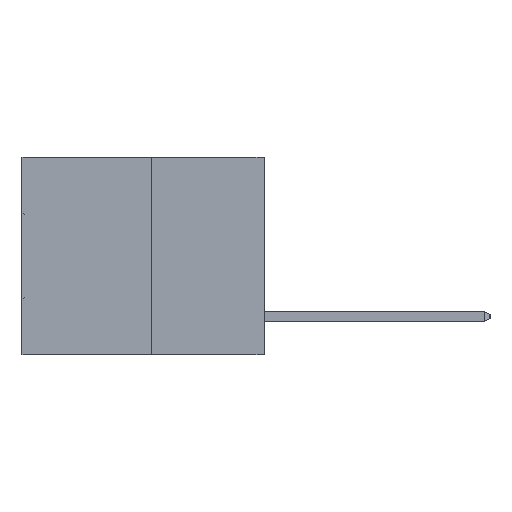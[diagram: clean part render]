
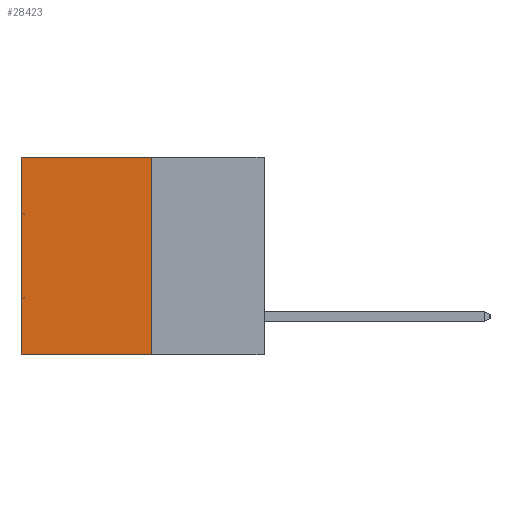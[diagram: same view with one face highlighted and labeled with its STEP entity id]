
A CAD part, left-side view. The second image highlights one B-rep face of the part: STEP entity #28423.
In plain terms, the highlighted planar face has unit normal (-1, 0, 0).
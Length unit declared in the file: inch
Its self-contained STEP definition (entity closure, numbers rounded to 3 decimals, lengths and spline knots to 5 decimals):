
#1631 = ORIENTED_EDGE ( 'NONE', *, *, #28231, .F. ) ;
#2117 = VERTEX_POINT ( 'NONE', #7423 ) ;
#2486 = CARTESIAN_POINT ( 'NONE',  ( 0.3165, 0.6, 0. ) ) ;
#2549 = CARTESIAN_POINT ( 'NONE',  ( 0.3165, 0.28, -0.49 ) ) ;
#2918 = CARTESIAN_POINT ( 'NONE',  ( 0.3165, 0.28, -0.49 ) ) ;
#4837 = LINE ( 'NONE', #11628, #22365 ) ;
#5639 = ORIENTED_EDGE ( 'NONE', *, *, #14806, .T. ) ;
#6487 = CARTESIAN_POINT ( 'NONE',  ( 0.3165, 0.6, -0.49 ) ) ;
#7120 = AXIS2_PLACEMENT_3D ( 'NONE', #2549, #17815, #20364 ) ;
#7423 = CARTESIAN_POINT ( 'NONE',  ( 0.3165, 0.28, 0. ) ) ;
#8020 = EDGE_CURVE ( 'NONE', #2117, #30886, #32022, .T. ) ;
#8221 = VERTEX_POINT ( 'NONE', #16242 ) ;
#10411 = DIRECTION ( 'NONE',  ( 0., 1., 0. ) ) ;
#11049 = VECTOR ( 'NONE', #24077, 39.37008 ) ;
#11628 = CARTESIAN_POINT ( 'NONE',  ( 0.3165, 0.28, -0.49 ) ) ;
#12649 = LINE ( 'NONE', #6487, #11049 ) ;
#14806 = EDGE_CURVE ( 'NONE', #30886, #14814, #12649, .T. ) ;
#14814 = VERTEX_POINT ( 'NONE', #26418 ) ;
#15567 = CARTESIAN_POINT ( 'NONE',  ( 0.3165, 0.28, 0. ) ) ;
#16242 = CARTESIAN_POINT ( 'NONE',  ( 0.3165, 0.28, -0.49 ) ) ;
#17815 = DIRECTION ( 'NONE',  ( 1., 0., 0. ) ) ;
#20364 = DIRECTION ( 'NONE',  ( 0., 0., -1. ) ) ;
#22033 = ORIENTED_EDGE ( 'NONE', *, *, #8020, .T. ) ;
#22213 = VECTOR ( 'NONE', #27823, 39.37008 ) ;
#22365 = VECTOR ( 'NONE', #28964, 39.37008 ) ;
#23432 = ORIENTED_EDGE ( 'NONE', *, *, #31177, .F. ) ;
#24077 = DIRECTION ( 'NONE',  ( 0., 0., -1. ) ) ;
#24204 = FACE_OUTER_BOUND ( 'NONE', #24785, .T. ) ;
#24785 = EDGE_LOOP ( 'NONE', ( #5639, #23432, #1631, #22033 ) ) ;
#25276 = VECTOR ( 'NONE', #10411, 39.37008 ) ;
#26418 = CARTESIAN_POINT ( 'NONE',  ( 0.3165, 0.6, -0.49 ) ) ;
#27823 = DIRECTION ( 'NONE',  ( 0., 0., -1. ) ) ;
#28001 = PLANE ( 'NONE',  #7120 ) ;
#28231 = EDGE_CURVE ( 'NONE', #2117, #8221, #28559, .T. ) ;
#28423 = ADVANCED_FACE ( 'NONE', ( #24204 ), #28001, .F. ) ;
#28559 = LINE ( 'NONE', #2918, #22213 ) ;
#28964 = DIRECTION ( 'NONE',  ( 0., 1., 0. ) ) ;
#30886 = VERTEX_POINT ( 'NONE', #2486 ) ;
#31177 = EDGE_CURVE ( 'NONE', #8221, #14814, #4837, .T. ) ;
#32022 = LINE ( 'NONE', #15567, #25276 ) ;
